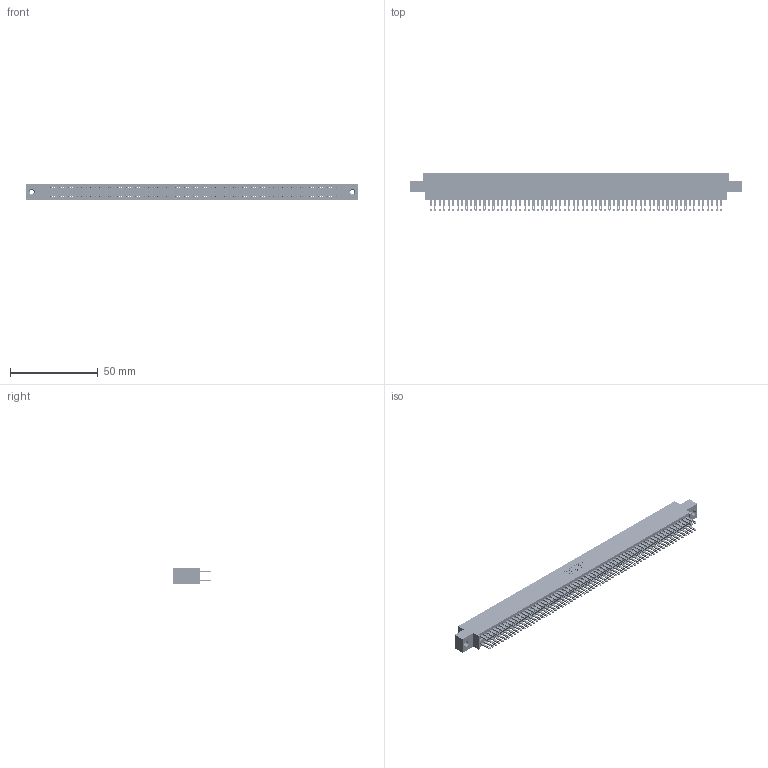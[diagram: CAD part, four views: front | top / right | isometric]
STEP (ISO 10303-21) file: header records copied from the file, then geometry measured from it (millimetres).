
FILE_DESCRIPTION (( 'STEP AP203' ), '1' );
FILE_NAME ('895-132-500-807.STEP', '2020-10-13T17:42:12', ( '' ), ( '' ), 'SwSTEP 2.0', 'SolidWorks 2020', '' );
FILE_SCHEMA (( 'CONFIG_CONTROL_DESIGN' ));
Length unit declared in the file: inch
Products named in the file (4): 345-292-001_345-293-100; 895-132-500-807; 845 Part_0.170 Offset - 0.156 Dia-TI; 345-250-001_345-250-005-103
Assembly tree (135 placements, depth 2):
  895-132-500-807
    845 Part_0.170 Offset - 0.156 Dia-TI
    345-292-001_345-293-100  x132
    345-250-001_345-250-005-103  x2
Bounding box: 188.85 x 21.51 x 9.4 mm (x, y, z)
Volume: 18844.2 mm3; surface area: 29837.4 mm2
Topology: 135 solids, 135 shells, 6262 faces, 19101 edges, 12726 vertices
Faces by surface type: plane 3680, cylinder 2566, cone 12, torus 4
Entity records: 49802 total; most frequent: CARTESIAN_POINT 8307, ORIENTED_EDGE 8234, DIRECTION 7323, EDGE_CURVE 4117, VECTOR 3697, LINE 3697, VERTEX_POINT 2740, AXIS2_PLACEMENT_3D 1813
